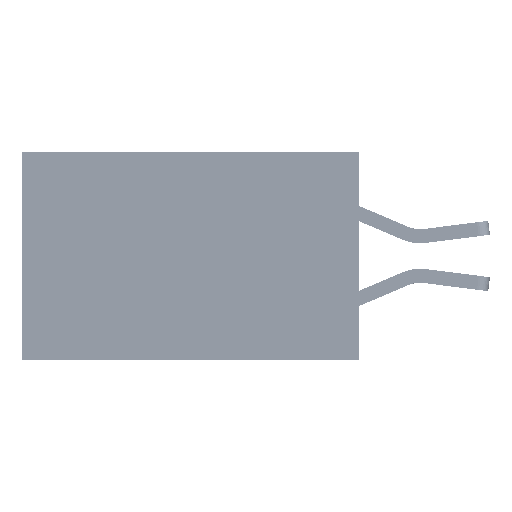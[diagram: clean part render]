
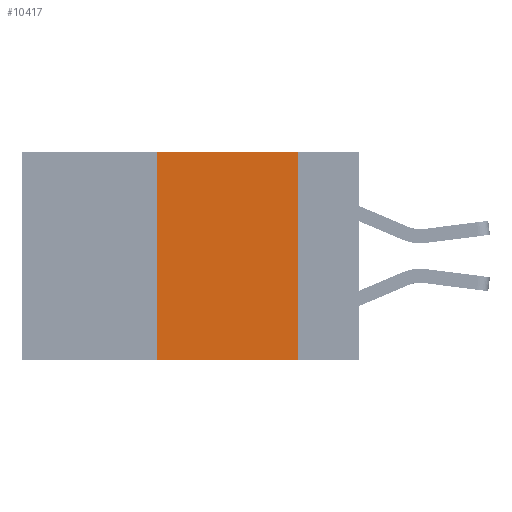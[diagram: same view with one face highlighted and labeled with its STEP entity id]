
A CAD part, left-side view. The second image highlights one B-rep face of the part: STEP entity #10417.
In plain terms, the highlighted planar face has unit normal (-1, 0, 0).
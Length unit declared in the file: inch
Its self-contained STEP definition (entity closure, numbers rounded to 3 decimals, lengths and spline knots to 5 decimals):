
#659 = CARTESIAN_POINT ( 'NONE',  ( 0., 0.36, -0.37 ) ) ;
#1431 = ORIENTED_EDGE ( 'NONE', *, *, #11302, .F. ) ;
#4623 = CARTESIAN_POINT ( 'NONE',  ( 0., 0.6, -0.37 ) ) ;
#5881 = CARTESIAN_POINT ( 'NONE',  ( 0., 0.11, 0. ) ) ;
#6977 = EDGE_LOOP ( 'NONE', ( #13900, #1431, #16033, #23213 ) ) ;
#7715 = DIRECTION ( 'NONE',  ( 0., -1., 0. ) ) ;
#8458 = VERTEX_POINT ( 'NONE', #5881 ) ;
#9647 = CARTESIAN_POINT ( 'NONE',  ( 0., 0.36, 0. ) ) ;
#10417 = ADVANCED_FACE ( 'NONE', ( #36352 ), #17821, .F. ) ;
#10726 = VECTOR ( 'NONE', #34269, 39.37008 ) ;
#11302 = EDGE_CURVE ( 'NONE', #26524, #8458, #21771, .T. ) ;
#11466 = EDGE_CURVE ( 'NONE', #21585, #34436, #16513, .T. ) ;
#11499 = DIRECTION ( 'NONE',  ( 1., 0., 0. ) ) ;
#12133 = DIRECTION ( 'NONE',  ( 0., 0., -1. ) ) ;
#13140 = CARTESIAN_POINT ( 'NONE',  ( 0., 0.36, 0. ) ) ;
#13900 = ORIENTED_EDGE ( 'NONE', *, *, #32252, .F. ) ;
#16033 = ORIENTED_EDGE ( 'NONE', *, *, #22120, .F. ) ;
#16513 = LINE ( 'NONE', #4623, #23710 ) ;
#17821 = PLANE ( 'NONE',  #20555 ) ;
#20159 = CARTESIAN_POINT ( 'NONE',  ( 0., 0.11, -0.37 ) ) ;
#20555 = AXIS2_PLACEMENT_3D ( 'NONE', #26851, #11499, #27114 ) ;
#21585 = VERTEX_POINT ( 'NONE', #659 ) ;
#21771 = LINE ( 'NONE', #31167, #10726 ) ;
#22120 = EDGE_CURVE ( 'NONE', #21585, #26524, #39590, .T. ) ;
#22617 = VECTOR ( 'NONE', #24439, 39.37008 ) ;
#23213 = ORIENTED_EDGE ( 'NONE', *, *, #11466, .T. ) ;
#23710 = VECTOR ( 'NONE', #7715, 39.37008 ) ;
#24439 = DIRECTION ( 'NONE',  ( 0., 0., 1. ) ) ;
#26172 = VECTOR ( 'NONE', #12133, 39.37008 ) ;
#26524 = VERTEX_POINT ( 'NONE', #13140 ) ;
#26851 = CARTESIAN_POINT ( 'NONE',  ( 0., 0.6, 0. ) ) ;
#27114 = DIRECTION ( 'NONE',  ( 0., 0., -1. ) ) ;
#31167 = CARTESIAN_POINT ( 'NONE',  ( 0., 0.6, 0. ) ) ;
#32252 = EDGE_CURVE ( 'NONE', #8458, #34436, #39257, .T. ) ;
#34269 = DIRECTION ( 'NONE',  ( 0., -1., 0. ) ) ;
#34436 = VERTEX_POINT ( 'NONE', #20159 ) ;
#36352 = FACE_OUTER_BOUND ( 'NONE', #6977, .T. ) ;
#36915 = CARTESIAN_POINT ( 'NONE',  ( 0., 0.11, 0. ) ) ;
#39257 = LINE ( 'NONE', #36915, #26172 ) ;
#39590 = LINE ( 'NONE', #9647, #22617 ) ;
